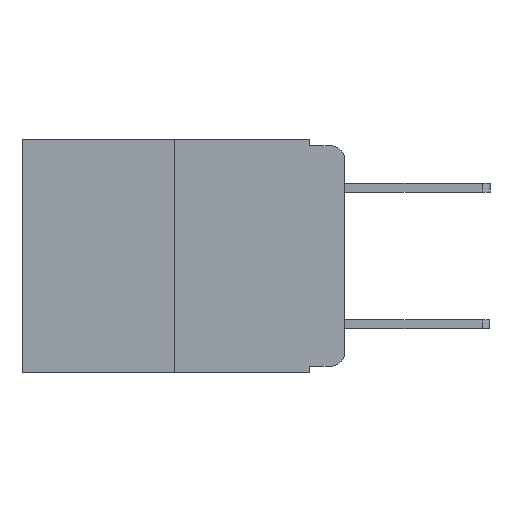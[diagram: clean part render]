
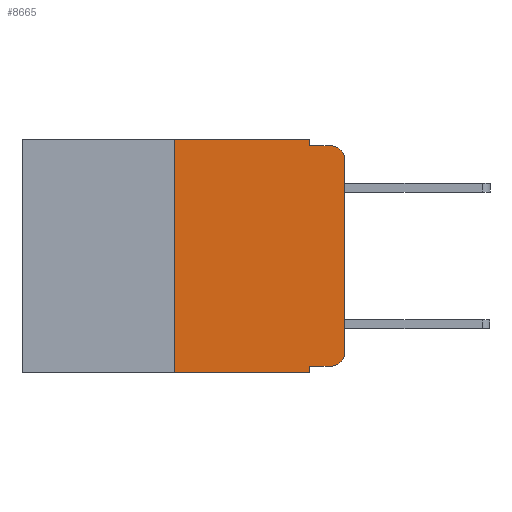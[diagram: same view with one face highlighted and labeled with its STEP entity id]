
A CAD part, left-side view. The second image highlights one B-rep face of the part: STEP entity #8665.
In plain terms, the highlighted planar face has unit normal (-1, 0, 0).
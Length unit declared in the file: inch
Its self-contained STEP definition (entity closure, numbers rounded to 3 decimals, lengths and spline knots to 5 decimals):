
#19 = EDGE_LOOP ( 'NONE', ( #2734, #2794, #2858, #2870, #2909, #2977, #2988, #3005, #3047, #3079 ) ) ;
#107 = LINE ( 'NONE', #8576, #6341 ) ;
#238 = VECTOR ( 'NONE', #6296, 39.37008 ) ;
#578 = CARTESIAN_POINT ( 'NONE',  ( 0., 0.25, 0. ) ) ;
#636 = AXIS2_PLACEMENT_3D ( 'NONE', #1635, #7353, #2492 ) ;
#712 = VERTEX_POINT ( 'NONE', #3892 ) ;
#803 = VERTEX_POINT ( 'NONE', #3266 ) ;
#822 = VERTEX_POINT ( 'NONE', #3093 ) ;
#844 = CARTESIAN_POINT ( 'NONE',  ( 0., 0.02, -0.03 ) ) ;
#1117 = VERTEX_POINT ( 'NONE', #4442 ) ;
#1285 = VECTOR ( 'NONE', #6082, 39.37008 ) ;
#1440 = VERTEX_POINT ( 'NONE', #3971 ) ;
#1635 = CARTESIAN_POINT ( 'NONE',  ( 0., 0.473, 0. ) ) ;
#1999 = AXIS2_PLACEMENT_3D ( 'NONE', #8486, #9976, #8817 ) ;
#2067 = CARTESIAN_POINT ( 'NONE',  ( 0., 0.473, -0.343 ) ) ;
#2089 = FACE_OUTER_BOUND ( 'NONE', #19, .T. ) ;
#2117 = LINE ( 'NONE', #3778, #6318 ) ;
#2281 = AXIS2_PLACEMENT_3D ( 'NONE', #844, #6335, #8081 ) ;
#2291 = EDGE_CURVE ( 'NONE', #2918, #2318, #2756, .T. ) ;
#2318 = VERTEX_POINT ( 'NONE', #7918 ) ;
#2492 = DIRECTION ( 'NONE',  ( 0., 0., -1. ) ) ;
#2541 = VERTEX_POINT ( 'NONE', #578 ) ;
#2734 = ORIENTED_EDGE ( 'NONE', *, *, #8752, .T. ) ;
#2756 = LINE ( 'NONE', #3070, #238 ) ;
#2794 = ORIENTED_EDGE ( 'NONE', *, *, #5720, .T. ) ;
#2858 = ORIENTED_EDGE ( 'NONE', *, *, #7669, .F. ) ;
#2870 = ORIENTED_EDGE ( 'NONE', *, *, #2291, .F. ) ;
#2881 = DIRECTION ( 'NONE',  ( 0., -1., 0. ) ) ;
#2909 = ORIENTED_EDGE ( 'NONE', *, *, #5659, .F. ) ;
#2918 = VERTEX_POINT ( 'NONE', #5356 ) ;
#2956 = DIRECTION ( 'NONE',  ( 0., 0., 1. ) ) ;
#2977 = ORIENTED_EDGE ( 'NONE', *, *, #5051, .F. ) ;
#2978 = VERTEX_POINT ( 'NONE', #8649 ) ;
#2988 = ORIENTED_EDGE ( 'NONE', *, *, #6870, .T. ) ;
#3005 = ORIENTED_EDGE ( 'NONE', *, *, #5459, .F. ) ;
#3016 = LINE ( 'NONE', #6470, #5802 ) ;
#3047 = ORIENTED_EDGE ( 'NONE', *, *, #5701, .T. ) ;
#3070 = CARTESIAN_POINT ( 'NONE',  ( 0., 0.051, 0. ) ) ;
#3079 = ORIENTED_EDGE ( 'NONE', *, *, #5937, .T. ) ;
#3093 = CARTESIAN_POINT ( 'NONE',  ( 0., 0.02, -0.01 ) ) ;
#3138 = LINE ( 'NONE', #5041, #7220 ) ;
#3266 = CARTESIAN_POINT ( 'NONE',  ( 0., 0.25, -0.343 ) ) ;
#3778 = CARTESIAN_POINT ( 'NONE',  ( 0., 0.25, 0. ) ) ;
#3892 = CARTESIAN_POINT ( 'NONE',  ( 0., 0.051, -0.333 ) ) ;
#3971 = CARTESIAN_POINT ( 'NONE',  ( 0., 0.02, -0.333 ) ) ;
#3974 = CARTESIAN_POINT ( 'NONE',  ( 0., 0.051, 0. ) ) ;
#4108 = LINE ( 'NONE', #2067, #8072 ) ;
#4442 = CARTESIAN_POINT ( 'NONE',  ( 0., 0., -0.03 ) ) ;
#5041 = CARTESIAN_POINT ( 'NONE',  ( 0., 0.051, -0.01 ) ) ;
#5051 = EDGE_CURVE ( 'NONE', #803, #2541, #2117, .T. ) ;
#5061 = CARTESIAN_POINT ( 'NONE',  ( 0., 0., 0. ) ) ;
#5356 = CARTESIAN_POINT ( 'NONE',  ( 0., 0.051, 0. ) ) ;
#5459 = EDGE_CURVE ( 'NONE', #712, #9612, #7963, .T. ) ;
#5484 = VECTOR ( 'NONE', #6749, 39.37008 ) ;
#5659 = EDGE_CURVE ( 'NONE', #2541, #2918, #107, .T. ) ;
#5701 = EDGE_CURVE ( 'NONE', #712, #1440, #3016, .T. ) ;
#5720 = EDGE_CURVE ( 'NONE', #1117, #822, #7127, .T. ) ;
#5802 = VECTOR ( 'NONE', #8064, 39.37008 ) ;
#5937 = EDGE_CURVE ( 'NONE', #1440, #2978, #6902, .T. ) ;
#5944 = DIRECTION ( 'NONE',  ( 0., -1., 0. ) ) ;
#6082 = DIRECTION ( 'NONE',  ( 0., 0., -1. ) ) ;
#6296 = DIRECTION ( 'NONE',  ( 0., 0., -1. ) ) ;
#6318 = VECTOR ( 'NONE', #2956, 39.37008 ) ;
#6335 = DIRECTION ( 'NONE',  ( -1., 0., 0. ) ) ;
#6341 = VECTOR ( 'NONE', #6479, 39.37008 ) ;
#6470 = CARTESIAN_POINT ( 'NONE',  ( 0., 0.051, -0.333 ) ) ;
#6479 = DIRECTION ( 'NONE',  ( 0., -1., 0. ) ) ;
#6749 = DIRECTION ( 'NONE',  ( 0., 0., 1. ) ) ;
#6870 = EDGE_CURVE ( 'NONE', #803, #9612, #4108, .T. ) ;
#6902 = CIRCLE ( 'NONE', #1999, 0.02 ) ;
#7127 = CIRCLE ( 'NONE', #2281, 0.02 ) ;
#7220 = VECTOR ( 'NONE', #5944, 39.37008 ) ;
#7353 = DIRECTION ( 'NONE',  ( 1., 0., 0. ) ) ;
#7669 = EDGE_CURVE ( 'NONE', #2318, #822, #3138, .T. ) ;
#7918 = CARTESIAN_POINT ( 'NONE',  ( 0., 0.051, -0.01 ) ) ;
#7963 = LINE ( 'NONE', #3974, #1285 ) ;
#8064 = DIRECTION ( 'NONE',  ( 0., -1., 0. ) ) ;
#8072 = VECTOR ( 'NONE', #2881, 39.37008 ) ;
#8081 = DIRECTION ( 'NONE',  ( 0., 0., -1. ) ) ;
#8486 = CARTESIAN_POINT ( 'NONE',  ( 0., 0.02, -0.313 ) ) ;
#8576 = CARTESIAN_POINT ( 'NONE',  ( 0., 0.473, 0. ) ) ;
#8649 = CARTESIAN_POINT ( 'NONE',  ( 0., 0., -0.313 ) ) ;
#8665 = ADVANCED_FACE ( 'NONE', ( #2089 ), #10133, .F. ) ;
#8752 = EDGE_CURVE ( 'NONE', #2978, #1117, #9365, .T. ) ;
#8817 = DIRECTION ( 'NONE',  ( 0., 0., -1. ) ) ;
#9009 = CARTESIAN_POINT ( 'NONE',  ( 0., 0.051, -0.343 ) ) ;
#9365 = LINE ( 'NONE', #5061, #5484 ) ;
#9612 = VERTEX_POINT ( 'NONE', #9009 ) ;
#9976 = DIRECTION ( 'NONE',  ( -1., 0., 0. ) ) ;
#10133 = PLANE ( 'NONE',  #636 ) ;
